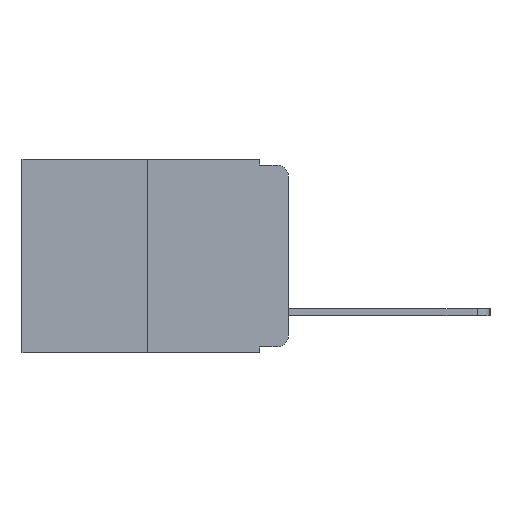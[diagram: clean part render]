
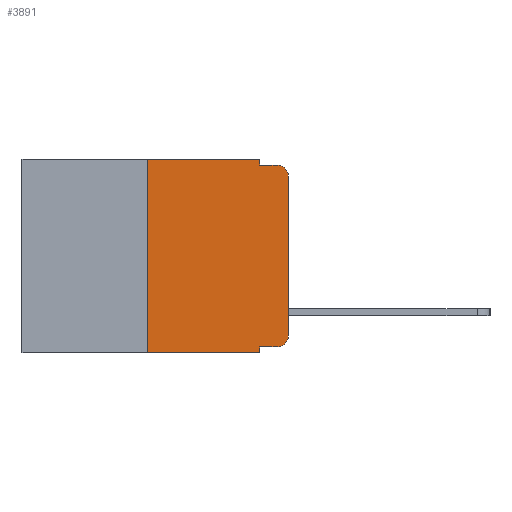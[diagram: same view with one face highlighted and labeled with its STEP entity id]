
A CAD part, left-side view. The second image highlights one B-rep face of the part: STEP entity #3891.
In plain terms, the highlighted planar face has unit normal (-1, 0, 0).
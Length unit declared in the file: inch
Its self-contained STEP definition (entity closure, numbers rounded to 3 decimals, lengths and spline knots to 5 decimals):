
#311 = EDGE_CURVE ( 'NONE', #5179, #8144, #5697, .T. ) ;
#520 = DIRECTION ( 'NONE',  ( -1., 0., 0. ) ) ;
#618 = VERTEX_POINT ( 'NONE', #3482 ) ;
#691 = AXIS2_PLACEMENT_3D ( 'NONE', #11621, #9450, #6013 ) ;
#796 = PLANE ( 'NONE',  #691 ) ;
#865 = ORIENTED_EDGE ( 'NONE', *, *, #1930, .T. ) ;
#918 = LINE ( 'NONE', #8069, #9888 ) ;
#932 = VECTOR ( 'NONE', #5155, 39.37008 ) ;
#1128 = ORIENTED_EDGE ( 'NONE', *, *, #2714, .T. ) ;
#1131 = EDGE_CURVE ( 'NONE', #8144, #6873, #7288, .T. ) ;
#1258 = DIRECTION ( 'NONE',  ( 0., -1., 0. ) ) ;
#1365 = ORIENTED_EDGE ( 'NONE', *, *, #12485, .T. ) ;
#1377 = ORIENTED_EDGE ( 'NONE', *, *, #311, .F. ) ;
#1739 = ORIENTED_EDGE ( 'NONE', *, *, #11791, .T. ) ;
#1796 = ORIENTED_EDGE ( 'NONE', *, *, #1131, .F. ) ;
#1842 = ORIENTED_EDGE ( 'NONE', *, *, #13159, .F. ) ;
#1930 = EDGE_CURVE ( 'NONE', #618, #6873, #5006, .T. ) ;
#1942 = CARTESIAN_POINT ( 'NONE',  ( 0., 0.02, -0.333 ) ) ;
#2681 = CARTESIAN_POINT ( 'NONE',  ( 0., 0.051, -0.343 ) ) ;
#2714 = EDGE_CURVE ( 'NONE', #8325, #618, #9421, .T. ) ;
#3062 = AXIS2_PLACEMENT_3D ( 'NONE', #12864, #12727, #12697 ) ;
#3187 = CARTESIAN_POINT ( 'NONE',  ( 0., 0.25, -0.343 ) ) ;
#3370 = AXIS2_PLACEMENT_3D ( 'NONE', #7429, #520, #8465 ) ;
#3426 = ORIENTED_EDGE ( 'NONE', *, *, #4036, .T. ) ;
#3482 = CARTESIAN_POINT ( 'NONE',  ( 0., 0., -0.03 ) ) ;
#3891 = ADVANCED_FACE ( 'NONE', ( #7738 ), #796, .F. ) ;
#4033 = CARTESIAN_POINT ( 'NONE',  ( 0., 0.051, 0. ) ) ;
#4036 = EDGE_CURVE ( 'NONE', #8604, #6093, #918, .T. ) ;
#4101 = LINE ( 'NONE', #4033, #932 ) ;
#4383 = CARTESIAN_POINT ( 'NONE',  ( 0., 0.02, -0.01 ) ) ;
#4422 = DIRECTION ( 'NONE',  ( 0., 0., -1. ) ) ;
#4429 = VERTEX_POINT ( 'NONE', #1942 ) ;
#4761 = CARTESIAN_POINT ( 'NONE',  ( 0., 0.473, 0. ) ) ;
#4914 = DIRECTION ( 'NONE',  ( 0., 0., 1. ) ) ;
#5006 = CIRCLE ( 'NONE', #3062, 0.02 ) ;
#5039 = VERTEX_POINT ( 'NONE', #10596 ) ;
#5155 = DIRECTION ( 'NONE',  ( 0., 0., -1. ) ) ;
#5179 = VERTEX_POINT ( 'NONE', #10476 ) ;
#5332 = VECTOR ( 'NONE', #4422, 39.37008 ) ;
#5697 = LINE ( 'NONE', #11012, #5332 ) ;
#5941 = EDGE_LOOP ( 'NONE', ( #1128, #865, #1796, #1377, #6118, #14090, #3426, #1842, #1365, #1739 ) ) ;
#6013 = DIRECTION ( 'NONE',  ( 0., 0., -1. ) ) ;
#6093 = VERTEX_POINT ( 'NONE', #2681 ) ;
#6118 = ORIENTED_EDGE ( 'NONE', *, *, #13736, .F. ) ;
#6873 = VERTEX_POINT ( 'NONE', #4383 ) ;
#7288 = LINE ( 'NONE', #10016, #12541 ) ;
#7406 = DIRECTION ( 'NONE',  ( 0., -1., 0. ) ) ;
#7429 = CARTESIAN_POINT ( 'NONE',  ( 0., 0.02, -0.313 ) ) ;
#7645 = DIRECTION ( 'NONE',  ( 0., -1., 0. ) ) ;
#7738 = FACE_OUTER_BOUND ( 'NONE', #5941, .T. ) ;
#7858 = CARTESIAN_POINT ( 'NONE',  ( 0., 0.051, -0.333 ) ) ;
#8069 = CARTESIAN_POINT ( 'NONE',  ( 0., 0.473, -0.343 ) ) ;
#8144 = VERTEX_POINT ( 'NONE', #10051 ) ;
#8325 = VERTEX_POINT ( 'NONE', #9248 ) ;
#8465 = DIRECTION ( 'NONE',  ( 0., 0., -1. ) ) ;
#8604 = VERTEX_POINT ( 'NONE', #3187 ) ;
#9248 = CARTESIAN_POINT ( 'NONE',  ( 0., 0., -0.313 ) ) ;
#9421 = LINE ( 'NONE', #9584, #12199 ) ;
#9450 = DIRECTION ( 'NONE',  ( 1., 0., 0. ) ) ;
#9584 = CARTESIAN_POINT ( 'NONE',  ( 0., 0., 0. ) ) ;
#9714 = CIRCLE ( 'NONE', #3370, 0.02 ) ;
#9735 = DIRECTION ( 'NONE',  ( 0., 0., 1. ) ) ;
#9885 = LINE ( 'NONE', #11340, #12646 ) ;
#9888 = VECTOR ( 'NONE', #7645, 39.37008 ) ;
#10016 = CARTESIAN_POINT ( 'NONE',  ( 0., 0.051, -0.01 ) ) ;
#10051 = CARTESIAN_POINT ( 'NONE',  ( 0., 0.051, -0.01 ) ) ;
#10052 = DIRECTION ( 'NONE',  ( 0., -1., 0. ) ) ;
#10476 = CARTESIAN_POINT ( 'NONE',  ( 0., 0.051, 0. ) ) ;
#10553 = LINE ( 'NONE', #4761, #10862 ) ;
#10596 = CARTESIAN_POINT ( 'NONE',  ( 0., 0.25, 0. ) ) ;
#10862 = VECTOR ( 'NONE', #1258, 39.37008 ) ;
#11012 = CARTESIAN_POINT ( 'NONE',  ( 0., 0.051, 0. ) ) ;
#11340 = CARTESIAN_POINT ( 'NONE',  ( 0., 0.25, 0. ) ) ;
#11504 = VERTEX_POINT ( 'NONE', #7858 ) ;
#11621 = CARTESIAN_POINT ( 'NONE',  ( 0., 0.473, 0. ) ) ;
#11791 = EDGE_CURVE ( 'NONE', #4429, #8325, #9714, .T. ) ;
#12199 = VECTOR ( 'NONE', #9735, 39.37008 ) ;
#12485 = EDGE_CURVE ( 'NONE', #11504, #4429, #12938, .T. ) ;
#12541 = VECTOR ( 'NONE', #10052, 39.37008 ) ;
#12646 = VECTOR ( 'NONE', #4914, 39.37008 ) ;
#12697 = DIRECTION ( 'NONE',  ( 0., 0., -1. ) ) ;
#12727 = DIRECTION ( 'NONE',  ( -1., 0., 0. ) ) ;
#12864 = CARTESIAN_POINT ( 'NONE',  ( 0., 0.02, -0.03 ) ) ;
#12938 = LINE ( 'NONE', #13629, #13248 ) ;
#13159 = EDGE_CURVE ( 'NONE', #11504, #6093, #4101, .T. ) ;
#13248 = VECTOR ( 'NONE', #7406, 39.37008 ) ;
#13629 = CARTESIAN_POINT ( 'NONE',  ( 0., 0.051, -0.333 ) ) ;
#13736 = EDGE_CURVE ( 'NONE', #5039, #5179, #10553, .T. ) ;
#13810 = EDGE_CURVE ( 'NONE', #8604, #5039, #9885, .T. ) ;
#14090 = ORIENTED_EDGE ( 'NONE', *, *, #13810, .F. ) ;
